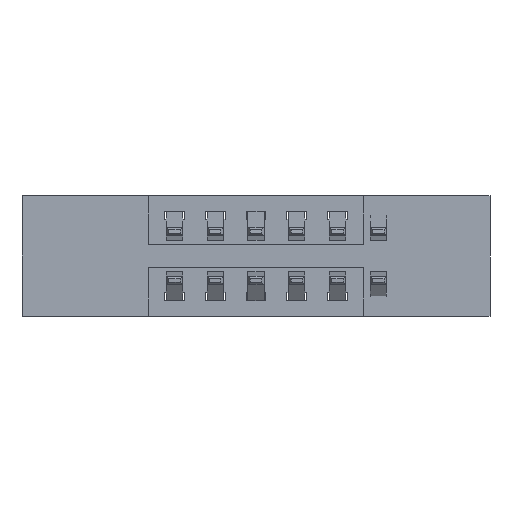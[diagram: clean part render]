
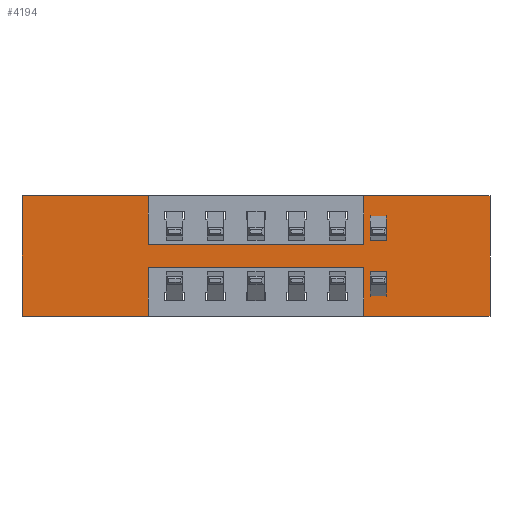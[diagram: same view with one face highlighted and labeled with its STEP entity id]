
A CAD part, front view. The second image highlights one B-rep face of the part: STEP entity #4194.
In plain terms, the highlighted planar face has unit normal (0, -1, 0).
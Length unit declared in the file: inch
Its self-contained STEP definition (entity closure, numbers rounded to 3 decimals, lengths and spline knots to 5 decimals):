
#130 = DIRECTION ( 'NONE',  ( -1., 0., 0. ) ) ;
#147 = ORIENTED_EDGE ( 'NONE', *, *, #8176, .F. ) ;
#200 = CARTESIAN_POINT ( 'NONE',  ( 0., 0., 0. ) ) ;
#260 = VECTOR ( 'NONE', #2654, 39.37008 ) ;
#267 = LINE ( 'NONE', #7874, #4002 ) ;
#442 = ORIENTED_EDGE ( 'NONE', *, *, #5832, .F. ) ;
#666 = CARTESIAN_POINT ( 'NONE',  ( 1.0475, 0., 0. ) ) ;
#753 = LINE ( 'NONE', #200, #3248 ) ;
#833 = ORIENTED_EDGE ( 'NONE', *, *, #6742, .F. ) ;
#860 = ORIENTED_EDGE ( 'NONE', *, *, #2515, .F. ) ;
#906 = DIRECTION ( 'NONE',  ( 0., -1., 0. ) ) ;
#1092 = VERTEX_POINT ( 'NONE', #8387 ) ;
#1119 = VERTEX_POINT ( 'NONE', #4410 ) ;
#1247 = CARTESIAN_POINT ( 'NONE',  ( 0.3875, 0., 0. ) ) ;
#1339 = LINE ( 'NONE', #5884, #260 ) ;
#1532 = CARTESIAN_POINT ( 'NONE',  ( 1.435, 0., 0. ) ) ;
#1595 = ORIENTED_EDGE ( 'NONE', *, *, #7354, .F. ) ;
#1625 = VECTOR ( 'NONE', #7183, 39.37008 ) ;
#1652 = DIRECTION ( 'NONE',  ( -1., 0., 0. ) ) ;
#1787 = ORIENTED_EDGE ( 'NONE', *, *, #7030, .F. ) ;
#1834 = DIRECTION ( 'NONE',  ( 1., 0., 0. ) ) ;
#1911 = VERTEX_POINT ( 'NONE', #6018 ) ;
#1914 = CARTESIAN_POINT ( 'NONE',  ( 0., 0., -0.37 ) ) ;
#1920 = LINE ( 'NONE', #4467, #7656 ) ;
#2124 = CARTESIAN_POINT ( 'NONE',  ( 0., 0., -0.37 ) ) ;
#2175 = CARTESIAN_POINT ( 'NONE',  ( 0.3875, 0., -0.37 ) ) ;
#2195 = LINE ( 'NONE', #1532, #3958 ) ;
#2509 = ORIENTED_EDGE ( 'NONE', *, *, #4539, .F. ) ;
#2515 = EDGE_CURVE ( 'NONE', #3428, #4417, #1920, .T. ) ;
#2571 = DIRECTION ( 'NONE',  ( -1., 0., 0. ) ) ;
#2654 = DIRECTION ( 'NONE',  ( 1., 0., 0. ) ) ;
#2699 = VERTEX_POINT ( 'NONE', #3072 ) ;
#2798 = CARTESIAN_POINT ( 'NONE',  ( 1.0475, 0., -0.37 ) ) ;
#2928 = LINE ( 'NONE', #2798, #3813 ) ;
#2934 = DIRECTION ( 'NONE',  ( 0., 0., -1. ) ) ;
#2953 = LINE ( 'NONE', #5547, #3046 ) ;
#2969 = CARTESIAN_POINT ( 'NONE',  ( 0.3875, 0., 0. ) ) ;
#3046 = VECTOR ( 'NONE', #1652, 39.37008 ) ;
#3072 = CARTESIAN_POINT ( 'NONE',  ( 1.0475, 0., -0.15 ) ) ;
#3184 = VECTOR ( 'NONE', #5953, 39.37008 ) ;
#3248 = VECTOR ( 'NONE', #6649, 39.37008 ) ;
#3428 = VERTEX_POINT ( 'NONE', #5792 ) ;
#3500 = FACE_OUTER_BOUND ( 'NONE', #8150, .T. ) ;
#3617 = CARTESIAN_POINT ( 'NONE',  ( 1.0475, 0., -0.37 ) ) ;
#3719 = ORIENTED_EDGE ( 'NONE', *, *, #7011, .F. ) ;
#3813 = VECTOR ( 'NONE', #7460, 39.37008 ) ;
#3864 = ORIENTED_EDGE ( 'NONE', *, *, #6168, .F. ) ;
#3958 = VECTOR ( 'NONE', #6160, 39.37008 ) ;
#4002 = VECTOR ( 'NONE', #6606, 39.37008 ) ;
#4097 = LINE ( 'NONE', #2175, #3184 ) ;
#4156 = LINE ( 'NONE', #666, #1625 ) ;
#4194 = ADVANCED_FACE ( 'NONE', ( #3500 ), #7367, .T. ) ;
#4376 = VECTOR ( 'NONE', #130, 39.37008 ) ;
#4410 = CARTESIAN_POINT ( 'NONE',  ( 1.0475, 0., -0.22 ) ) ;
#4417 = VERTEX_POINT ( 'NONE', #1914 ) ;
#4467 = CARTESIAN_POINT ( 'NONE',  ( 0., 0., -0.37 ) ) ;
#4490 = VECTOR ( 'NONE', #2934, 39.37008 ) ;
#4539 = EDGE_CURVE ( 'NONE', #4417, #6567, #753, .T. ) ;
#4561 = ORIENTED_EDGE ( 'NONE', *, *, #7343, .F. ) ;
#4952 = CARTESIAN_POINT ( 'NONE',  ( 0.3875, 0., -0.15 ) ) ;
#5057 = VERTEX_POINT ( 'NONE', #1247 ) ;
#5231 = VERTEX_POINT ( 'NONE', #7076 ) ;
#5468 = VECTOR ( 'NONE', #1834, 39.37008 ) ;
#5547 = CARTESIAN_POINT ( 'NONE',  ( 0.3875, 0., -0.22 ) ) ;
#5792 = CARTESIAN_POINT ( 'NONE',  ( 0.3875, 0., -0.37 ) ) ;
#5832 = EDGE_CURVE ( 'NONE', #5231, #6873, #7909, .T. ) ;
#5884 = CARTESIAN_POINT ( 'NONE',  ( 0., 0., 0. ) ) ;
#5953 = DIRECTION ( 'NONE',  ( 0., 0., -1. ) ) ;
#6018 = CARTESIAN_POINT ( 'NONE',  ( 0.3875, 0., -0.22 ) ) ;
#6160 = DIRECTION ( 'NONE',  ( 0., 0., -1. ) ) ;
#6168 = EDGE_CURVE ( 'NONE', #6567, #5057, #8029, .T. ) ;
#6567 = VERTEX_POINT ( 'NONE', #7736 ) ;
#6599 = VERTEX_POINT ( 'NONE', #7234 ) ;
#6606 = DIRECTION ( 'NONE',  ( 1., 0., 0. ) ) ;
#6649 = DIRECTION ( 'NONE',  ( 0., 0., 1. ) ) ;
#6742 = EDGE_CURVE ( 'NONE', #1119, #1911, #2953, .T. ) ;
#6761 = EDGE_CURVE ( 'NONE', #1911, #3428, #4097, .T. ) ;
#6832 = EDGE_CURVE ( 'NONE', #7910, #2699, #267, .T. ) ;
#6873 = VERTEX_POINT ( 'NONE', #3617 ) ;
#6911 = AXIS2_PLACEMENT_3D ( 'NONE', #7444, #906, #7996 ) ;
#7011 = EDGE_CURVE ( 'NONE', #6873, #1119, #2928, .T. ) ;
#7030 = EDGE_CURVE ( 'NONE', #6599, #5231, #2195, .T. ) ;
#7046 = ORIENTED_EDGE ( 'NONE', *, *, #6832, .F. ) ;
#7076 = CARTESIAN_POINT ( 'NONE',  ( 1.435, 0., -0.37 ) ) ;
#7183 = DIRECTION ( 'NONE',  ( 0., 0., 1. ) ) ;
#7234 = CARTESIAN_POINT ( 'NONE',  ( 1.435, 0., 0. ) ) ;
#7343 = EDGE_CURVE ( 'NONE', #2699, #1092, #4156, .T. ) ;
#7354 = EDGE_CURVE ( 'NONE', #1092, #6599, #1339, .T. ) ;
#7367 = PLANE ( 'NONE',  #6911 ) ;
#7444 = CARTESIAN_POINT ( 'NONE',  ( 0., 0., -0.37 ) ) ;
#7460 = DIRECTION ( 'NONE',  ( 0., 0., 1. ) ) ;
#7656 = VECTOR ( 'NONE', #2571, 39.37008 ) ;
#7665 = ORIENTED_EDGE ( 'NONE', *, *, #6761, .F. ) ;
#7736 = CARTESIAN_POINT ( 'NONE',  ( 0., 0., 0. ) ) ;
#7874 = CARTESIAN_POINT ( 'NONE',  ( 0.3875, 0., -0.15 ) ) ;
#7909 = LINE ( 'NONE', #2124, #4376 ) ;
#7910 = VERTEX_POINT ( 'NONE', #4952 ) ;
#7983 = LINE ( 'NONE', #2969, #4490 ) ;
#7996 = DIRECTION ( 'NONE',  ( 0., 0., -1. ) ) ;
#8029 = LINE ( 'NONE', #8207, #5468 ) ;
#8150 = EDGE_LOOP ( 'NONE', ( #7665, #833, #3719, #442, #1787, #1595, #4561, #7046, #147, #3864, #2509, #860 ) ) ;
#8176 = EDGE_CURVE ( 'NONE', #5057, #7910, #7983, .T. ) ;
#8207 = CARTESIAN_POINT ( 'NONE',  ( 0., 0., 0. ) ) ;
#8387 = CARTESIAN_POINT ( 'NONE',  ( 1.0475, 0., 0. ) ) ;
